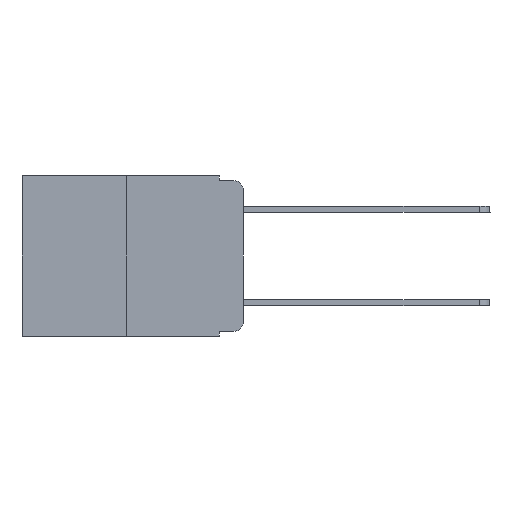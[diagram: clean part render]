
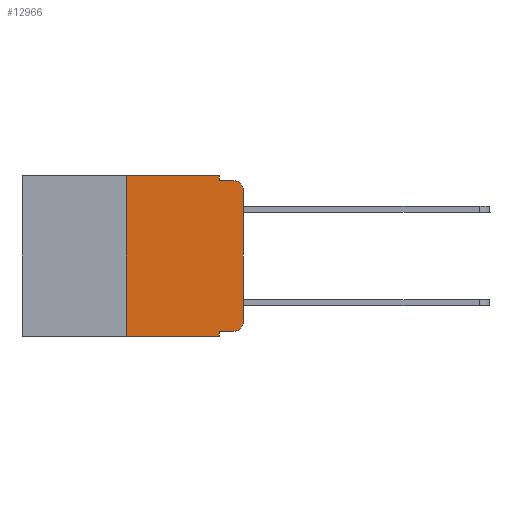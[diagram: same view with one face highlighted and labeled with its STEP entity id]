
A CAD part, left-side view. The second image highlights one B-rep face of the part: STEP entity #12966.
In plain terms, the highlighted planar face has unit normal (-1, 0, 0).
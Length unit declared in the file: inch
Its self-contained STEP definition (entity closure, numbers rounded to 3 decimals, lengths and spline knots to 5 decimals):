
#9 = LINE ( 'NONE', #10934, #7473 ) ;
#55 = AXIS2_PLACEMENT_3D ( 'NONE', #4487, #5894, #11502 ) ;
#209 = AXIS2_PLACEMENT_3D ( 'NONE', #10476, #6548, #16324 ) ;
#464 = CARTESIAN_POINT ( 'NONE',  ( 0., 0.051, -0.333 ) ) ;
#519 = VECTOR ( 'NONE', #11282, 39.37008 ) ;
#650 = ORIENTED_EDGE ( 'NONE', *, *, #13891, .T. ) ;
#838 = CARTESIAN_POINT ( 'NONE',  ( 0., 0.051, -0.343 ) ) ;
#986 = ORIENTED_EDGE ( 'NONE', *, *, #7717, .F. ) ;
#1078 = ORIENTED_EDGE ( 'NONE', *, *, #17918, .T. ) ;
#1111 = FACE_OUTER_BOUND ( 'NONE', #8594, .T. ) ;
#1985 = VECTOR ( 'NONE', #2489, 39.37008 ) ;
#2209 = DIRECTION ( 'NONE',  ( 0., 0., -1. ) ) ;
#2271 = ORIENTED_EDGE ( 'NONE', *, *, #12704, .F. ) ;
#2458 = VECTOR ( 'NONE', #7147, 39.37008 ) ;
#2489 = DIRECTION ( 'NONE',  ( 0., -1., 0. ) ) ;
#2549 = VERTEX_POINT ( 'NONE', #8008 ) ;
#3135 = VERTEX_POINT ( 'NONE', #8207 ) ;
#3161 = ORIENTED_EDGE ( 'NONE', *, *, #17243, .T. ) ;
#3519 = CARTESIAN_POINT ( 'NONE',  ( 0., 0.051, -0.01 ) ) ;
#3802 = CARTESIAN_POINT ( 'NONE',  ( 0., 0., 0. ) ) ;
#4316 = LINE ( 'NONE', #9884, #519 ) ;
#4487 = CARTESIAN_POINT ( 'NONE',  ( 0., 0.473, 0. ) ) ;
#4498 = EDGE_CURVE ( 'NONE', #3135, #17225, #4316, .T. ) ;
#5643 = CARTESIAN_POINT ( 'NONE',  ( 0., 0.051, -0.333 ) ) ;
#5894 = DIRECTION ( 'NONE',  ( 1., 0., 0. ) ) ;
#5895 = ORIENTED_EDGE ( 'NONE', *, *, #7572, .F. ) ;
#5985 = VERTEX_POINT ( 'NONE', #9920 ) ;
#6227 = CARTESIAN_POINT ( 'NONE',  ( 0., 0.25, 0. ) ) ;
#6548 = DIRECTION ( 'NONE',  ( -1., 0., 0. ) ) ;
#6911 = VERTEX_POINT ( 'NONE', #5643 ) ;
#7147 = DIRECTION ( 'NONE',  ( 0., 0., -1. ) ) ;
#7473 = VECTOR ( 'NONE', #10814, 39.37008 ) ;
#7572 = EDGE_CURVE ( 'NONE', #17225, #17347, #14257, .T. ) ;
#7717 = EDGE_CURVE ( 'NONE', #6911, #14932, #14052, .T. ) ;
#8008 = CARTESIAN_POINT ( 'NONE',  ( 0., 0., -0.03 ) ) ;
#8022 = CARTESIAN_POINT ( 'NONE',  ( 0., 0.02, -0.03 ) ) ;
#8207 = CARTESIAN_POINT ( 'NONE',  ( 0., 0.051, 0. ) ) ;
#8594 = EDGE_LOOP ( 'NONE', ( #650, #1078, #5895, #9728, #2271, #10640, #16269, #986, #14205, #3161 ) ) ;
#8802 = CIRCLE ( 'NONE', #16220, 0.02 ) ;
#8860 = DIRECTION ( 'NONE',  ( 0., 0., 1. ) ) ;
#8924 = VERTEX_POINT ( 'NONE', #10919 ) ;
#9048 = CARTESIAN_POINT ( 'NONE',  ( 0., 0., -0.313 ) ) ;
#9110 = CARTESIAN_POINT ( 'NONE',  ( 0., 0.25, 0. ) ) ;
#9728 = ORIENTED_EDGE ( 'NONE', *, *, #4498, .F. ) ;
#9884 = CARTESIAN_POINT ( 'NONE',  ( 0., 0.051, 0. ) ) ;
#9920 = CARTESIAN_POINT ( 'NONE',  ( 0., 0.25, -0.343 ) ) ;
#10126 = CIRCLE ( 'NONE', #209, 0.02 ) ;
#10154 = PLANE ( 'NONE',  #55 ) ;
#10476 = CARTESIAN_POINT ( 'NONE',  ( 0., 0.02, -0.313 ) ) ;
#10498 = VERTEX_POINT ( 'NONE', #6227 ) ;
#10640 = ORIENTED_EDGE ( 'NONE', *, *, #17782, .F. ) ;
#10700 = VECTOR ( 'NONE', #15926, 39.37008 ) ;
#10814 = DIRECTION ( 'NONE',  ( 0., -1., 0. ) ) ;
#10919 = CARTESIAN_POINT ( 'NONE',  ( 0., 0.02, -0.333 ) ) ;
#10934 = CARTESIAN_POINT ( 'NONE',  ( 0., 0.473, 0. ) ) ;
#10945 = DIRECTION ( 'NONE',  ( 0., 0., 1. ) ) ;
#11282 = DIRECTION ( 'NONE',  ( 0., 0., -1. ) ) ;
#11502 = DIRECTION ( 'NONE',  ( 0., 0., -1. ) ) ;
#12704 = EDGE_CURVE ( 'NONE', #10498, #3135, #9, .T. ) ;
#12966 = ADVANCED_FACE ( 'NONE', ( #1111 ), #10154, .F. ) ;
#13198 = LINE ( 'NONE', #13577, #17820 ) ;
#13577 = CARTESIAN_POINT ( 'NONE',  ( 0., 0.473, -0.343 ) ) ;
#13811 = CARTESIAN_POINT ( 'NONE',  ( 0., 0.02, -0.01 ) ) ;
#13891 = EDGE_CURVE ( 'NONE', #14868, #2549, #17070, .T. ) ;
#13920 = CARTESIAN_POINT ( 'NONE',  ( 0., 0.051, 0. ) ) ;
#14052 = LINE ( 'NONE', #13920, #2458 ) ;
#14205 = ORIENTED_EDGE ( 'NONE', *, *, #14296, .T. ) ;
#14257 = LINE ( 'NONE', #17961, #1985 ) ;
#14296 = EDGE_CURVE ( 'NONE', #6911, #8924, #17490, .T. ) ;
#14720 = VECTOR ( 'NONE', #8860, 39.37008 ) ;
#14868 = VERTEX_POINT ( 'NONE', #9048 ) ;
#14886 = DIRECTION ( 'NONE',  ( -1., 0., 0. ) ) ;
#14932 = VERTEX_POINT ( 'NONE', #838 ) ;
#14972 = DIRECTION ( 'NONE',  ( 0., -1., 0. ) ) ;
#15926 = DIRECTION ( 'NONE',  ( 0., -1., 0. ) ) ;
#16208 = VECTOR ( 'NONE', #10945, 39.37008 ) ;
#16220 = AXIS2_PLACEMENT_3D ( 'NONE', #8022, #14886, #2209 ) ;
#16269 = ORIENTED_EDGE ( 'NONE', *, *, #17325, .T. ) ;
#16324 = DIRECTION ( 'NONE',  ( 0., 0., -1. ) ) ;
#16955 = LINE ( 'NONE', #9110, #14720 ) ;
#17070 = LINE ( 'NONE', #3802, #16208 ) ;
#17225 = VERTEX_POINT ( 'NONE', #3519 ) ;
#17243 = EDGE_CURVE ( 'NONE', #8924, #14868, #10126, .T. ) ;
#17325 = EDGE_CURVE ( 'NONE', #5985, #14932, #13198, .T. ) ;
#17347 = VERTEX_POINT ( 'NONE', #13811 ) ;
#17490 = LINE ( 'NONE', #464, #10700 ) ;
#17782 = EDGE_CURVE ( 'NONE', #5985, #10498, #16955, .T. ) ;
#17820 = VECTOR ( 'NONE', #14972, 39.37008 ) ;
#17918 = EDGE_CURVE ( 'NONE', #2549, #17347, #8802, .T. ) ;
#17961 = CARTESIAN_POINT ( 'NONE',  ( 0., 0.051, -0.01 ) ) ;
